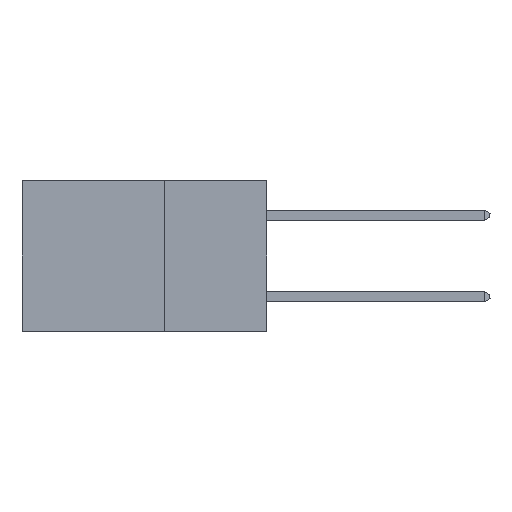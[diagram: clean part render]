
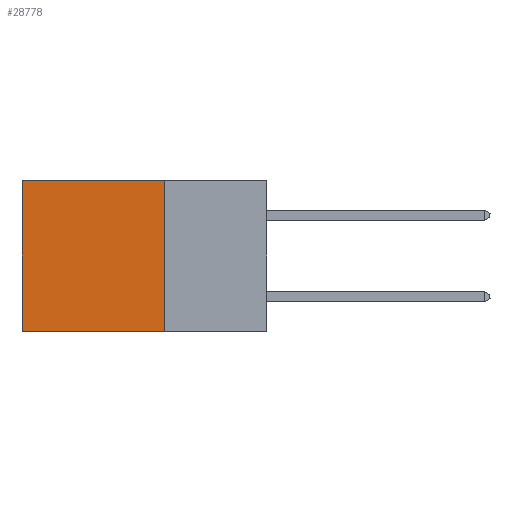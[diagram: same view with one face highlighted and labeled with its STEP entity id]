
A CAD part, left-side view. The second image highlights one B-rep face of the part: STEP entity #28778.
In plain terms, the highlighted planar face has unit normal (-1, 0, 0).
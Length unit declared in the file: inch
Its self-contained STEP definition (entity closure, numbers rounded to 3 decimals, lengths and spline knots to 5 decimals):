
#217 = DIRECTION ( 'NONE',  ( 0., 0., -1. ) ) ;
#615 = CARTESIAN_POINT ( 'NONE',  ( 0.2875, 0.25, 0. ) ) ;
#876 = LINE ( 'NONE', #22635, #25098 ) ;
#1044 = CARTESIAN_POINT ( 'NONE',  ( 0.2875, 0.25, -0.37 ) ) ;
#2535 = CARTESIAN_POINT ( 'NONE',  ( 0.2875, 0.25, 0. ) ) ;
#2817 = AXIS2_PLACEMENT_3D ( 'NONE', #9423, #11856, #217 ) ;
#3047 = CARTESIAN_POINT ( 'NONE',  ( 0.2875, 0.25, -0.37 ) ) ;
#3502 = CARTESIAN_POINT ( 'NONE',  ( 0.2875, 0.6, 0. ) ) ;
#4860 = VECTOR ( 'NONE', #9992, 39.37008 ) ;
#9423 = CARTESIAN_POINT ( 'NONE',  ( 0.2875, 0.25, 0. ) ) ;
#9720 = VECTOR ( 'NONE', #12915, 39.37008 ) ;
#9905 = PLANE ( 'NONE',  #2817 ) ;
#9992 = DIRECTION ( 'NONE',  ( 0., 1., 0. ) ) ;
#10016 = EDGE_CURVE ( 'NONE', #26487, #18705, #876, .T. ) ;
#10844 = VERTEX_POINT ( 'NONE', #3502 ) ;
#11629 = FACE_OUTER_BOUND ( 'NONE', #15224, .T. ) ;
#11856 = DIRECTION ( 'NONE',  ( 1., 0., 0. ) ) ;
#12611 = ORIENTED_EDGE ( 'NONE', *, *, #19679, .T. ) ;
#12903 = DIRECTION ( 'NONE',  ( 0., 1., 0. ) ) ;
#12915 = DIRECTION ( 'NONE',  ( 0., 0., -1. ) ) ;
#14275 = VECTOR ( 'NONE', #12903, 39.37008 ) ;
#14440 = LINE ( 'NONE', #24425, #9720 ) ;
#15224 = EDGE_LOOP ( 'NONE', ( #12611, #21211, #19513, #27549 ) ) ;
#15680 = DIRECTION ( 'NONE',  ( 0., 0., -1. ) ) ;
#17032 = EDGE_CURVE ( 'NONE', #18705, #21845, #21557, .T. ) ;
#18705 = VERTEX_POINT ( 'NONE', #1044 ) ;
#19513 = ORIENTED_EDGE ( 'NONE', *, *, #10016, .F. ) ;
#19679 = EDGE_CURVE ( 'NONE', #10844, #21845, #14440, .T. ) ;
#21211 = ORIENTED_EDGE ( 'NONE', *, *, #17032, .F. ) ;
#21557 = LINE ( 'NONE', #3047, #14275 ) ;
#21635 = LINE ( 'NONE', #615, #4860 ) ;
#21845 = VERTEX_POINT ( 'NONE', #22952 ) ;
#22635 = CARTESIAN_POINT ( 'NONE',  ( 0.2875, 0.25, 0. ) ) ;
#22952 = CARTESIAN_POINT ( 'NONE',  ( 0.2875, 0.6, -0.37 ) ) ;
#24425 = CARTESIAN_POINT ( 'NONE',  ( 0.2875, 0.6, 0. ) ) ;
#25098 = VECTOR ( 'NONE', #15680, 39.37008 ) ;
#26487 = VERTEX_POINT ( 'NONE', #2535 ) ;
#26965 = EDGE_CURVE ( 'NONE', #26487, #10844, #21635, .T. ) ;
#27549 = ORIENTED_EDGE ( 'NONE', *, *, #26965, .T. ) ;
#28778 = ADVANCED_FACE ( 'NONE', ( #11629 ), #9905, .F. ) ;
